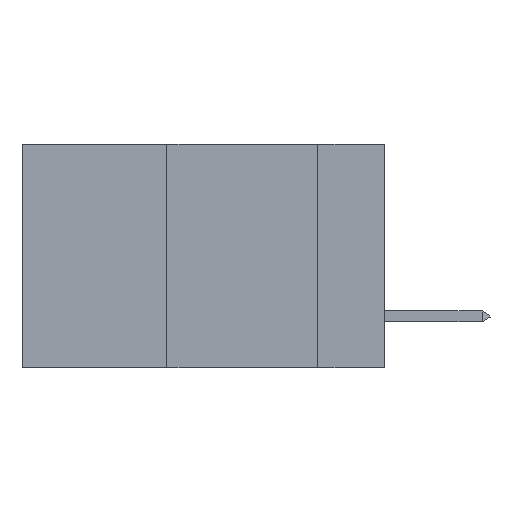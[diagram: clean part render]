
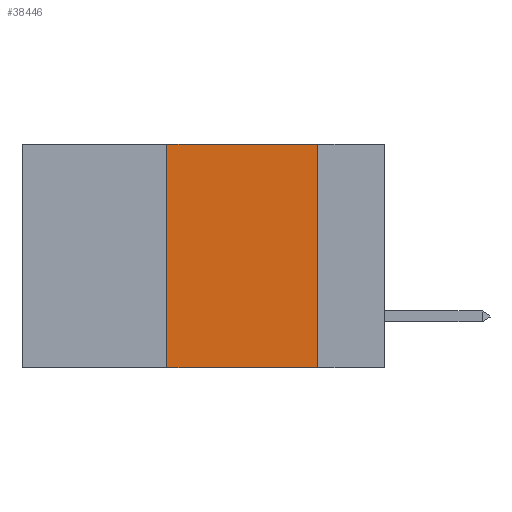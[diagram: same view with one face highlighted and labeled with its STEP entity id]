
A CAD part, left-side view. The second image highlights one B-rep face of the part: STEP entity #38446.
In plain terms, the highlighted planar face has unit normal (-1, 0, 0).
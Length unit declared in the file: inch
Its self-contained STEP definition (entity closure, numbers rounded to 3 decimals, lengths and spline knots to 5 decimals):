
#818 = EDGE_CURVE ( 'NONE', #5210, #19187, #8713, .T. ) ;
#1926 = VECTOR ( 'NONE', #32950, 39.37008 ) ;
#3347 = CARTESIAN_POINT ( 'NONE',  ( 0., 0.36, 0. ) ) ;
#3691 = VERTEX_POINT ( 'NONE', #14161 ) ;
#4077 = EDGE_CURVE ( 'NONE', #26707, #5210, #11405, .T. ) ;
#5210 = VERTEX_POINT ( 'NONE', #7078 ) ;
#5526 = PLANE ( 'NONE',  #22549 ) ;
#5573 = ORIENTED_EDGE ( 'NONE', *, *, #4077, .F. ) ;
#5663 = DIRECTION ( 'NONE',  ( 0., 0., -1. ) ) ;
#6322 = LINE ( 'NONE', #10580, #1926 ) ;
#7078 = CARTESIAN_POINT ( 'NONE',  ( 0., 0.36, 0. ) ) ;
#8713 = LINE ( 'NONE', #27915, #26803 ) ;
#9070 = CARTESIAN_POINT ( 'NONE',  ( 0., 0.11, 0. ) ) ;
#9890 = VECTOR ( 'NONE', #24939, 39.37008 ) ;
#10580 = CARTESIAN_POINT ( 'NONE',  ( 0., 0.6, -0.37 ) ) ;
#10983 = VECTOR ( 'NONE', #36936, 39.37008 ) ;
#11405 = LINE ( 'NONE', #3347, #9890 ) ;
#13334 = CARTESIAN_POINT ( 'NONE',  ( 0., 0.11, 0. ) ) ;
#14161 = CARTESIAN_POINT ( 'NONE',  ( 0., 0.11, -0.37 ) ) ;
#19187 = VERTEX_POINT ( 'NONE', #13334 ) ;
#20535 = EDGE_CURVE ( 'NONE', #19187, #3691, #21271, .T. ) ;
#20950 = ORIENTED_EDGE ( 'NONE', *, *, #24043, .T. ) ;
#21212 = DIRECTION ( 'NONE',  ( 1., 0., 0. ) ) ;
#21271 = LINE ( 'NONE', #9070, #10983 ) ;
#22549 = AXIS2_PLACEMENT_3D ( 'NONE', #39517, #21212, #5663 ) ;
#23167 = CARTESIAN_POINT ( 'NONE',  ( 0., 0.36, -0.37 ) ) ;
#24043 = EDGE_CURVE ( 'NONE', #26707, #3691, #6322, .T. ) ;
#24259 = ORIENTED_EDGE ( 'NONE', *, *, #20535, .F. ) ;
#24939 = DIRECTION ( 'NONE',  ( 0., 0., 1. ) ) ;
#26367 = ORIENTED_EDGE ( 'NONE', *, *, #818, .F. ) ;
#26707 = VERTEX_POINT ( 'NONE', #23167 ) ;
#26803 = VECTOR ( 'NONE', #30785, 39.37008 ) ;
#27915 = CARTESIAN_POINT ( 'NONE',  ( 0., 0.6, 0. ) ) ;
#29582 = FACE_OUTER_BOUND ( 'NONE', #39859, .T. ) ;
#30785 = DIRECTION ( 'NONE',  ( 0., -1., 0. ) ) ;
#32950 = DIRECTION ( 'NONE',  ( 0., -1., 0. ) ) ;
#36936 = DIRECTION ( 'NONE',  ( 0., 0., -1. ) ) ;
#38446 = ADVANCED_FACE ( 'NONE', ( #29582 ), #5526, .F. ) ;
#39517 = CARTESIAN_POINT ( 'NONE',  ( 0., 0.6, 0. ) ) ;
#39859 = EDGE_LOOP ( 'NONE', ( #24259, #26367, #5573, #20950 ) ) ;
